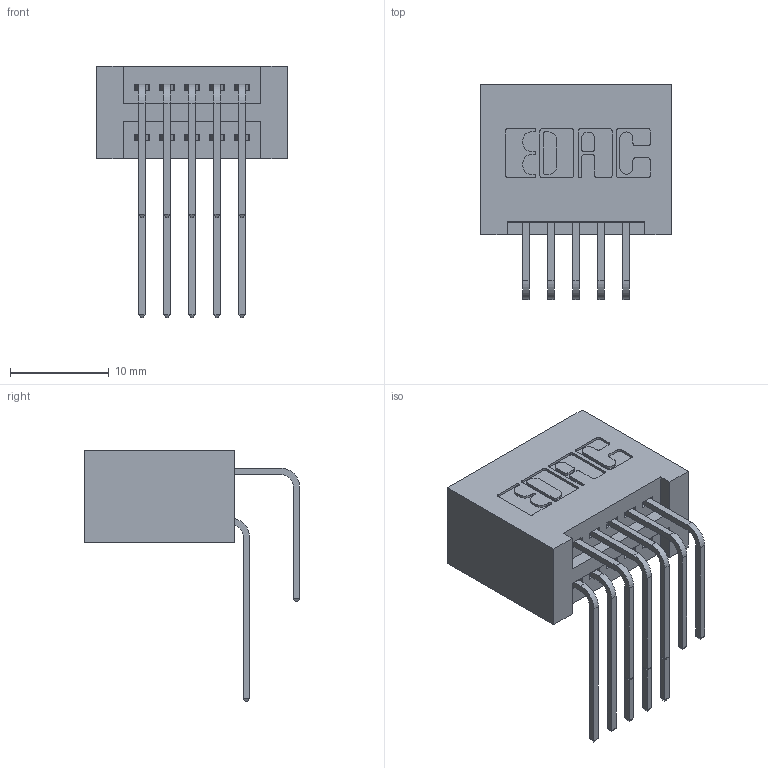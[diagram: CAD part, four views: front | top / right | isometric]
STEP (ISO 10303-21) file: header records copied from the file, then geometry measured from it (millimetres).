
FILE_DESCRIPTION (( 'STEP AP203' ), '1' );
FILE_NAME ('395-010-558-201.STEP', '2019-10-15T12:08:58', ( '' ), ( '' ), 'SwSTEP 2.0', 'SolidWorks 2016', '' );
FILE_SCHEMA (( 'CONFIG_CONTROL_DESIGN' ));
Length unit declared in the file: inch
Products named in the file (4): 345 Part_No Mounting Lugs; 345-292-001_558 559 Tail - 1; 345-292-001_558 Tail - 2; 395-010-558-201
Assembly tree (11 placements, depth 2):
  395-010-558-201
    345 Part_No Mounting Lugs
    345-292-001_558 559 Tail - 1  x5
    345-292-001_558 Tail - 2  x5
Bounding box: 19.3 x 21.83 x 25.53 mm (x, y, z)
Volume: 2205.4 mm3; surface area: 3117.8 mm2
Topology: 11 solids, 11 shells, 638 faces, 1867 edges, 1230 vertices
Faces by surface type: plane 426, cylinder 212
Entity records: 10279 total; most frequent: CARTESIAN_POINT 1803, ORIENTED_EDGE 1686, DIRECTION 1603, EDGE_CURVE 843, LINE 659, VECTOR 659, VERTEX_POINT 558, AXIS2_PLACEMENT_3D 472
